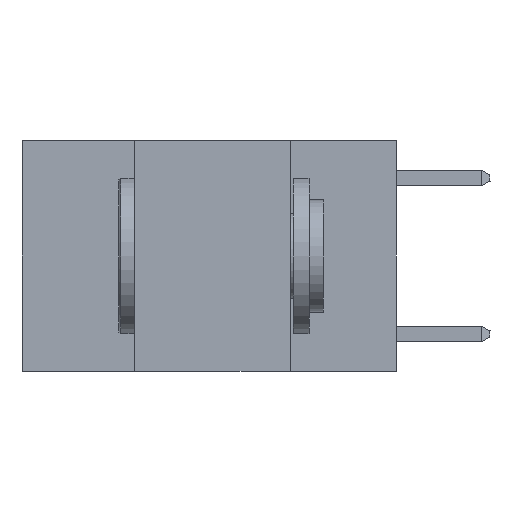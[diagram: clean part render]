
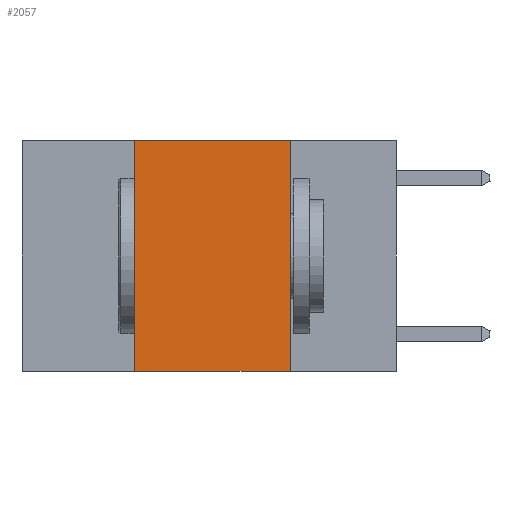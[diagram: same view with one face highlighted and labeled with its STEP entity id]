
A CAD part, left-side view. The second image highlights one B-rep face of the part: STEP entity #2057.
In plain terms, the highlighted planar face has unit normal (-1, 0, 0).
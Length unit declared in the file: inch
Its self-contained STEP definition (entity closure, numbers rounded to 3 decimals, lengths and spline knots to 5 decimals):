
#1314 = CARTESIAN_POINT ( 'NONE',  ( 0., 0.17, 0. ) ) ;
#1350 = EDGE_LOOP ( 'NONE', ( #8775, #4751, #3220, #12860 ) ) ;
#2057 = ADVANCED_FACE ( 'NONE', ( #12017 ), #2755, .F. ) ;
#2110 = VECTOR ( 'NONE', #6329, 39.37008 ) ;
#2278 = VERTEX_POINT ( 'NONE', #4009 ) ;
#2699 = DIRECTION ( 'NONE',  ( 1., 0., 0. ) ) ;
#2755 = PLANE ( 'NONE',  #9122 ) ;
#3220 = ORIENTED_EDGE ( 'NONE', *, *, #3352, .F. ) ;
#3352 = EDGE_CURVE ( 'NONE', #12050, #2278, #9595, .T. ) ;
#3851 = CARTESIAN_POINT ( 'NONE',  ( 0., 0.6, 0. ) ) ;
#4009 = CARTESIAN_POINT ( 'NONE',  ( 0., 0.42, 0. ) ) ;
#4590 = CARTESIAN_POINT ( 'NONE',  ( 0., 0.17, 0. ) ) ;
#4751 = ORIENTED_EDGE ( 'NONE', *, *, #13431, .F. ) ;
#4805 = CARTESIAN_POINT ( 'NONE',  ( 0., 0.6, 0. ) ) ;
#4905 = CARTESIAN_POINT ( 'NONE',  ( 0., 0.42, -0.37 ) ) ;
#5449 = VECTOR ( 'NONE', #8810, 39.37008 ) ;
#5635 = VECTOR ( 'NONE', #10494, 39.37008 ) ;
#5769 = VECTOR ( 'NONE', #12389, 39.37008 ) ;
#5831 = DIRECTION ( 'NONE',  ( 0., 0., -1. ) ) ;
#6265 = CARTESIAN_POINT ( 'NONE',  ( 0., 0.6, -0.37 ) ) ;
#6290 = CARTESIAN_POINT ( 'NONE',  ( 0., 0.42, 0. ) ) ;
#6329 = DIRECTION ( 'NONE',  ( 0., -1., 0. ) ) ;
#7284 = VERTEX_POINT ( 'NONE', #1314 ) ;
#7954 = LINE ( 'NONE', #3851, #5769 ) ;
#8775 = ORIENTED_EDGE ( 'NONE', *, *, #11018, .F. ) ;
#8810 = DIRECTION ( 'NONE',  ( 0., 0., -1. ) ) ;
#9122 = AXIS2_PLACEMENT_3D ( 'NONE', #4805, #2699, #5831 ) ;
#9331 = VERTEX_POINT ( 'NONE', #11240 ) ;
#9595 = LINE ( 'NONE', #6290, #5635 ) ;
#9825 = LINE ( 'NONE', #4590, #5449 ) ;
#10494 = DIRECTION ( 'NONE',  ( 0., 0., 1. ) ) ;
#10874 = EDGE_CURVE ( 'NONE', #12050, #9331, #11485, .T. ) ;
#11018 = EDGE_CURVE ( 'NONE', #7284, #9331, #9825, .T. ) ;
#11240 = CARTESIAN_POINT ( 'NONE',  ( 0., 0.17, -0.37 ) ) ;
#11485 = LINE ( 'NONE', #6265, #2110 ) ;
#12017 = FACE_OUTER_BOUND ( 'NONE', #1350, .T. ) ;
#12050 = VERTEX_POINT ( 'NONE', #4905 ) ;
#12389 = DIRECTION ( 'NONE',  ( 0., -1., 0. ) ) ;
#12860 = ORIENTED_EDGE ( 'NONE', *, *, #10874, .T. ) ;
#13431 = EDGE_CURVE ( 'NONE', #2278, #7284, #7954, .T. ) ;
